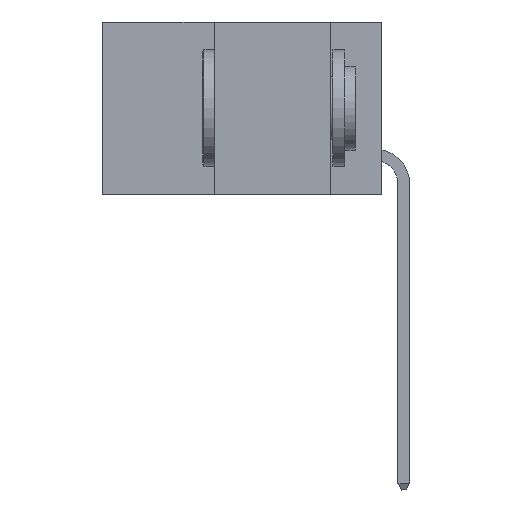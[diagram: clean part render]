
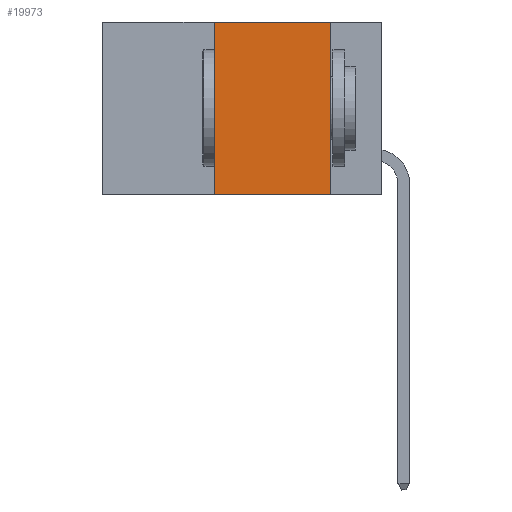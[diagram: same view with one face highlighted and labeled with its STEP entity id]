
A CAD part, left-side view. The second image highlights one B-rep face of the part: STEP entity #19973.
In plain terms, the highlighted planar face has unit normal (-1, 0, 0).
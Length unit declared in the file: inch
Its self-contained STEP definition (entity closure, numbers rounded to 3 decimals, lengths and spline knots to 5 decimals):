
#1007 = DIRECTION ( 'NONE',  ( 0., -1., 0. ) ) ;
#1023 = VECTOR ( 'NONE', #1007, 39.37008 ) ;
#1822 = EDGE_CURVE ( 'NONE', #7127, #14043, #18300, .T. ) ;
#2665 = DIRECTION ( 'NONE',  ( 0., 0., -1. ) ) ;
#2874 = EDGE_CURVE ( 'NONE', #20062, #5314, #10034, .T. ) ;
#3520 = EDGE_CURVE ( 'NONE', #7127, #20062, #10511, .T. ) ;
#4014 = DIRECTION ( 'NONE',  ( 0., 0., 1. ) ) ;
#4021 = CARTESIAN_POINT ( 'NONE',  ( 0., 0.6, 0. ) ) ;
#4272 = VECTOR ( 'NONE', #11404, 39.37008 ) ;
#4423 = FACE_OUTER_BOUND ( 'NONE', #8697, .T. ) ;
#5314 = VERTEX_POINT ( 'NONE', #6969 ) ;
#6037 = CARTESIAN_POINT ( 'NONE',  ( 0., 0.6, -0.37 ) ) ;
#6282 = LINE ( 'NONE', #11357, #18175 ) ;
#6969 = CARTESIAN_POINT ( 'NONE',  ( 0., 0.11, 0. ) ) ;
#7127 = VERTEX_POINT ( 'NONE', #19163 ) ;
#8616 = ORIENTED_EDGE ( 'NONE', *, *, #2874, .F. ) ;
#8697 = EDGE_LOOP ( 'NONE', ( #21922, #8616, #12724, #15164 ) ) ;
#9196 = CARTESIAN_POINT ( 'NONE',  ( 0., 0.36, 0. ) ) ;
#9203 = DIRECTION ( 'NONE',  ( 0., 0., -1. ) ) ;
#10034 = LINE ( 'NONE', #14470, #1023 ) ;
#10511 = LINE ( 'NONE', #9196, #11813 ) ;
#10517 = AXIS2_PLACEMENT_3D ( 'NONE', #4021, #14344, #9203 ) ;
#10660 = EDGE_CURVE ( 'NONE', #5314, #14043, #6282, .T. ) ;
#11357 = CARTESIAN_POINT ( 'NONE',  ( 0., 0.11, 0. ) ) ;
#11404 = DIRECTION ( 'NONE',  ( 0., -1., 0. ) ) ;
#11813 = VECTOR ( 'NONE', #4014, 39.37008 ) ;
#12724 = ORIENTED_EDGE ( 'NONE', *, *, #3520, .F. ) ;
#14043 = VERTEX_POINT ( 'NONE', #21989 ) ;
#14344 = DIRECTION ( 'NONE',  ( 1., 0., 0. ) ) ;
#14470 = CARTESIAN_POINT ( 'NONE',  ( 0., 0.6, 0. ) ) ;
#15164 = ORIENTED_EDGE ( 'NONE', *, *, #1822, .T. ) ;
#18175 = VECTOR ( 'NONE', #2665, 39.37008 ) ;
#18300 = LINE ( 'NONE', #6037, #4272 ) ;
#19163 = CARTESIAN_POINT ( 'NONE',  ( 0., 0.36, -0.37 ) ) ;
#19350 = PLANE ( 'NONE',  #10517 ) ;
#19973 = ADVANCED_FACE ( 'NONE', ( #4423 ), #19350, .F. ) ;
#20062 = VERTEX_POINT ( 'NONE', #21240 ) ;
#21240 = CARTESIAN_POINT ( 'NONE',  ( 0., 0.36, 0. ) ) ;
#21922 = ORIENTED_EDGE ( 'NONE', *, *, #10660, .F. ) ;
#21989 = CARTESIAN_POINT ( 'NONE',  ( 0., 0.11, -0.37 ) ) ;
